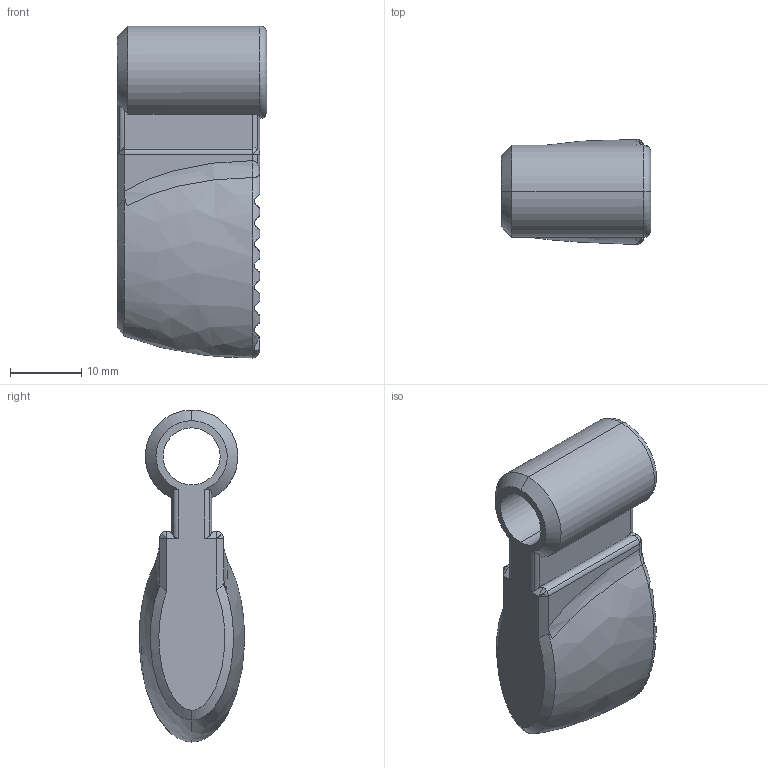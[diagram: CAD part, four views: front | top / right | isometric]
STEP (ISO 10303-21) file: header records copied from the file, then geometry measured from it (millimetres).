
FILE_DESCRIPTION(('STEP AP214'),'1');
FILE_NAME('Mod9 Charging Handle Final.stp','2020-09-28T22:46:15',(' '),(' '),'Spatial InterOp 3D',' ',' ');
FILE_SCHEMA(('AUTOMOTIVE_DESIGN { 1 0 10303 214 1 1 1 1 }'));
Length unit declared in the file: metre
Products named in the file (1): ASM Body
Bounding box: 21 x 14.74 x 46.57 mm (x, y, z)
Volume: 8310.2 mm3; surface area: 3556 mm2
Topology: 1 solids, 1 shells, 194 faces, 519 edges, 333 vertices
Faces by surface type: plane 147, cylinder 24, bspline 11, cone 6, sphere 4, torus 2
Entity records: 7055 total; most frequent: CARTESIAN_POINT 2334, ORIENTED_EDGE 1026, DIRECTION 886, EDGE_CURVE 513, LINE 348, VECTOR 348, VERTEX_POINT 333, AXIS2_PLACEMENT_3D 269
